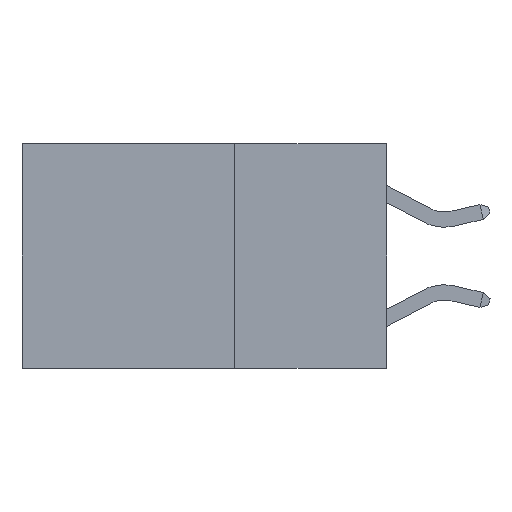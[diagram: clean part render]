
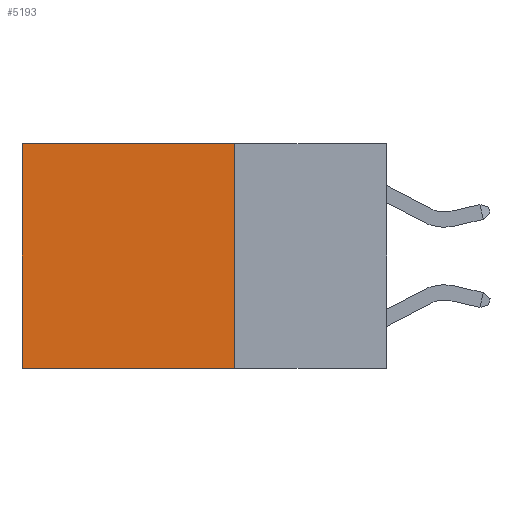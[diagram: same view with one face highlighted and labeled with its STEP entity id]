
A CAD part, left-side view. The second image highlights one B-rep face of the part: STEP entity #5193.
In plain terms, the highlighted planar face has unit normal (-1, 0, 0).
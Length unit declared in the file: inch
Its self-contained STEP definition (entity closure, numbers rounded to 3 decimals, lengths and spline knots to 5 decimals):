
#55 = DIRECTION ( 'NONE',  ( 0., 0., -1. ) ) ;
#177 = CARTESIAN_POINT ( 'NONE',  ( 0.2625, 0.25, 0. ) ) ;
#219 = VERTEX_POINT ( 'NONE', #4602 ) ;
#742 = PLANE ( 'NONE',  #5442 ) ;
#944 = VECTOR ( 'NONE', #4479, 39.37008 ) ;
#1303 = EDGE_CURVE ( 'NONE', #5879, #219, #1649, .T. ) ;
#1613 = CARTESIAN_POINT ( 'NONE',  ( 0.2625, 0.25, 0. ) ) ;
#1649 = LINE ( 'NONE', #4952, #8015 ) ;
#1787 = LINE ( 'NONE', #7594, #3767 ) ;
#1894 = CARTESIAN_POINT ( 'NONE',  ( 0.2625, 0.6, 0. ) ) ;
#2009 = VERTEX_POINT ( 'NONE', #4231 ) ;
#2164 = ORIENTED_EDGE ( 'NONE', *, *, #5051, .F. ) ;
#2179 = FACE_OUTER_BOUND ( 'NONE', #4921, .T. ) ;
#2247 = DIRECTION ( 'NONE',  ( 0., 0., -1. ) ) ;
#2622 = LINE ( 'NONE', #3397, #4017 ) ;
#3397 = CARTESIAN_POINT ( 'NONE',  ( 0.2625, 0.25, -0.37 ) ) ;
#3746 = DIRECTION ( 'NONE',  ( 0., 1., 0. ) ) ;
#3767 = VECTOR ( 'NONE', #3746, 39.37008 ) ;
#4017 = VECTOR ( 'NONE', #5231, 39.37008 ) ;
#4231 = CARTESIAN_POINT ( 'NONE',  ( 0.2625, 0.25, -0.37 ) ) ;
#4479 = DIRECTION ( 'NONE',  ( 0., 0., -1. ) ) ;
#4602 = CARTESIAN_POINT ( 'NONE',  ( 0.2625, 0.6, -0.37 ) ) ;
#4615 = LINE ( 'NONE', #6453, #944 ) ;
#4921 = EDGE_LOOP ( 'NONE', ( #6882, #6100, #2164, #5399 ) ) ;
#4952 = CARTESIAN_POINT ( 'NONE',  ( 0.2625, 0.6, 0. ) ) ;
#5051 = EDGE_CURVE ( 'NONE', #7161, #2009, #4615, .T. ) ;
#5193 = ADVANCED_FACE ( 'NONE', ( #2179 ), #742, .F. ) ;
#5231 = DIRECTION ( 'NONE',  ( 0., 1., 0. ) ) ;
#5399 = ORIENTED_EDGE ( 'NONE', *, *, #6688, .T. ) ;
#5442 = AXIS2_PLACEMENT_3D ( 'NONE', #177, #6044, #55 ) ;
#5499 = EDGE_CURVE ( 'NONE', #2009, #219, #2622, .T. ) ;
#5879 = VERTEX_POINT ( 'NONE', #1894 ) ;
#6044 = DIRECTION ( 'NONE',  ( 1., 0., 0. ) ) ;
#6100 = ORIENTED_EDGE ( 'NONE', *, *, #5499, .F. ) ;
#6453 = CARTESIAN_POINT ( 'NONE',  ( 0.2625, 0.25, 0. ) ) ;
#6688 = EDGE_CURVE ( 'NONE', #7161, #5879, #1787, .T. ) ;
#6882 = ORIENTED_EDGE ( 'NONE', *, *, #1303, .T. ) ;
#7161 = VERTEX_POINT ( 'NONE', #1613 ) ;
#7594 = CARTESIAN_POINT ( 'NONE',  ( 0.2625, 0.25, 0. ) ) ;
#8015 = VECTOR ( 'NONE', #2247, 39.37008 ) ;
